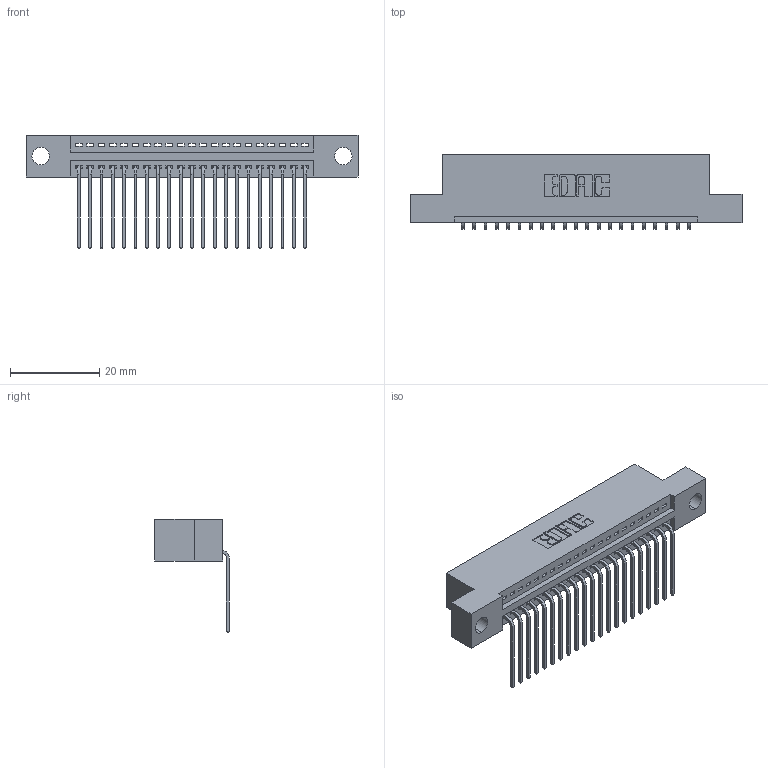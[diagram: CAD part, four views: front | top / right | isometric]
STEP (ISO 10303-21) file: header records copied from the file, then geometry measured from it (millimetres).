
FILE_DESCRIPTION (( 'STEP AP203' ), '1' );
FILE_NAME ('345-021-559-104.STEP', '2021-05-26T14:23:42', ( '' ), ( '' ), 'SwSTEP 2.0', 'SolidWorks 2020', '' );
FILE_SCHEMA (( 'CONFIG_CONTROL_DESIGN' ));
Length unit declared in the file: inch
Products named in the file (3): 345-021-559-104; 345 Part_Flush Mounting Lugs - 0.156 Dia-TI; 345-292-001_558 559 Tail - 1
Assembly tree (22 placements, depth 2):
  345-021-559-104
    345 Part_Flush Mounting Lugs - 0.156 Dia-TI
    345-292-001_558 559 Tail - 1  x21
Bounding box: 74.55 x 16.75 x 25.53 mm (x, y, z)
Volume: 6872.7 mm3; surface area: 9101.4 mm2
Topology: 22 solids, 22 shells, 1400 faces, 4199 edges, 2770 vertices
Faces by surface type: plane 976, cylinder 424
Entity records: 19135 total; most frequent: CARTESIAN_POINT 3325, ORIENTED_EDGE 3278, DIRECTION 2933, EDGE_CURVE 1639, VECTOR 1423, LINE 1423, VERTEX_POINT 1090, AXIS2_PLACEMENT_3D 755
